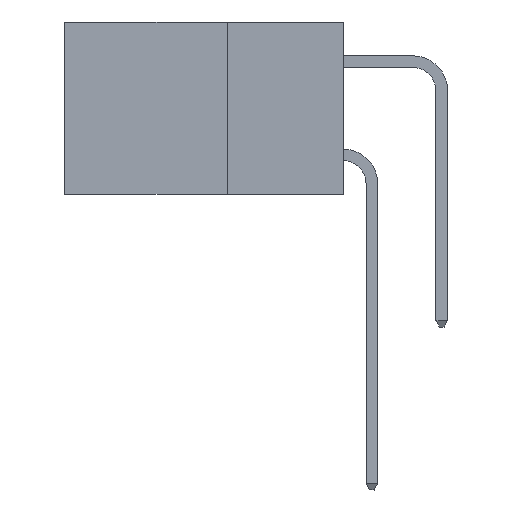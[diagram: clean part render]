
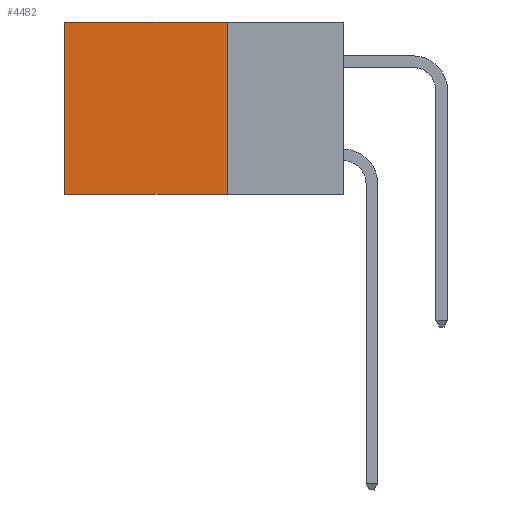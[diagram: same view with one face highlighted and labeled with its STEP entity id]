
A CAD part, left-side view. The second image highlights one B-rep face of the part: STEP entity #4482.
In plain terms, the highlighted planar face has unit normal (-1, 0, 0).
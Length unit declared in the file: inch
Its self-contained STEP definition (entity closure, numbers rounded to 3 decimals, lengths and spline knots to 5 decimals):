
#703 = AXIS2_PLACEMENT_3D ( 'NONE', #20007, #11170, #19586 ) ;
#2091 = VERTEX_POINT ( 'NONE', #11999 ) ;
#2284 = DIRECTION ( 'NONE',  ( 0., 0., -1. ) ) ;
#2630 = DIRECTION ( 'NONE',  ( 0., 0., -1. ) ) ;
#2911 = CARTESIAN_POINT ( 'NONE',  ( 0.2615, 0.6, -0.37 ) ) ;
#4482 = ADVANCED_FACE ( 'NONE', ( #8917 ), #11450, .F. ) ;
#4498 = LINE ( 'NONE', #15200, #6623 ) ;
#6623 = VECTOR ( 'NONE', #12691, 39.37008 ) ;
#7296 = ORIENTED_EDGE ( 'NONE', *, *, #15081, .T. ) ;
#8917 = FACE_OUTER_BOUND ( 'NONE', #14951, .T. ) ;
#11170 = DIRECTION ( 'NONE',  ( 1., 0., 0. ) ) ;
#11193 = VECTOR ( 'NONE', #2284, 39.37008 ) ;
#11321 = EDGE_CURVE ( 'NONE', #15821, #26724, #18303, .T. ) ;
#11450 = PLANE ( 'NONE',  #703 ) ;
#11989 = CARTESIAN_POINT ( 'NONE',  ( 0.2615, 0.6, 0. ) ) ;
#11999 = CARTESIAN_POINT ( 'NONE',  ( 0.2615, 0.6, -0.37 ) ) ;
#12131 = ORIENTED_EDGE ( 'NONE', *, *, #21848, .F. ) ;
#12209 = ORIENTED_EDGE ( 'NONE', *, *, #23496, .F. ) ;
#12691 = DIRECTION ( 'NONE',  ( 0., 1., 0. ) ) ;
#14951 = EDGE_LOOP ( 'NONE', ( #7296, #12131, #12209, #16980 ) ) ;
#15081 = EDGE_CURVE ( 'NONE', #26724, #2091, #17703, .T. ) ;
#15200 = CARTESIAN_POINT ( 'NONE',  ( 0.2615, 0.25, -0.37 ) ) ;
#15461 = CARTESIAN_POINT ( 'NONE',  ( 0.2615, 0.25, -0.37 ) ) ;
#15521 = LINE ( 'NONE', #24092, #11193 ) ;
#15821 = VERTEX_POINT ( 'NONE', #19306 ) ;
#16177 = DIRECTION ( 'NONE',  ( 0., 1., 0. ) ) ;
#16980 = ORIENTED_EDGE ( 'NONE', *, *, #11321, .T. ) ;
#17703 = LINE ( 'NONE', #2911, #23503 ) ;
#18303 = LINE ( 'NONE', #22666, #18950 ) ;
#18950 = VECTOR ( 'NONE', #16177, 39.37008 ) ;
#19306 = CARTESIAN_POINT ( 'NONE',  ( 0.2615, 0.25, 0. ) ) ;
#19586 = DIRECTION ( 'NONE',  ( 0., 0., -1. ) ) ;
#20007 = CARTESIAN_POINT ( 'NONE',  ( 0.2615, 0.25, -0.37 ) ) ;
#21848 = EDGE_CURVE ( 'NONE', #27103, #2091, #4498, .T. ) ;
#22666 = CARTESIAN_POINT ( 'NONE',  ( 0.2615, 0.25, 0. ) ) ;
#23496 = EDGE_CURVE ( 'NONE', #15821, #27103, #15521, .T. ) ;
#23503 = VECTOR ( 'NONE', #2630, 39.37008 ) ;
#24092 = CARTESIAN_POINT ( 'NONE',  ( 0.2615, 0.25, -0.37 ) ) ;
#26724 = VERTEX_POINT ( 'NONE', #11989 ) ;
#27103 = VERTEX_POINT ( 'NONE', #15461 ) ;
